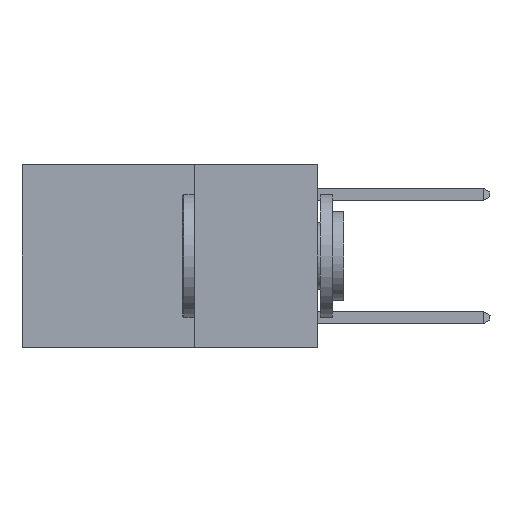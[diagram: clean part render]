
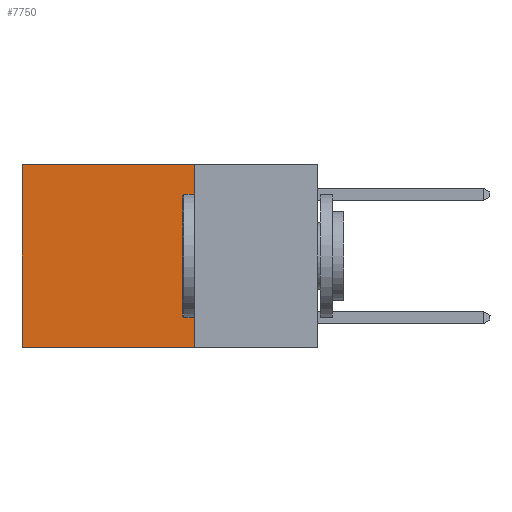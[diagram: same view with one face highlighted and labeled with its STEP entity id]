
A CAD part, left-side view. The second image highlights one B-rep face of the part: STEP entity #7750.
In plain terms, the highlighted planar face has unit normal (-1, 0, 0).
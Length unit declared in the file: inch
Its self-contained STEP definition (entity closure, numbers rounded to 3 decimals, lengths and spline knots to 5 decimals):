
#570 = EDGE_CURVE ( 'NONE', #6980, #10879, #2409, .T. ) ;
#599 = LINE ( 'NONE', #3156, #6562 ) ;
#1293 = DIRECTION ( 'NONE',  ( 0., 0., -1. ) ) ;
#1350 = VECTOR ( 'NONE', #5822, 39.37008 ) ;
#1358 = CARTESIAN_POINT ( 'NONE',  ( 0.2625, 0.25, 0. ) ) ;
#1656 = EDGE_CURVE ( 'NONE', #10879, #11398, #599, .T. ) ;
#2409 = LINE ( 'NONE', #2677, #4765 ) ;
#2545 = AXIS2_PLACEMENT_3D ( 'NONE', #5964, #5924, #1293 ) ;
#2677 = CARTESIAN_POINT ( 'NONE',  ( 0.2625, 0.25, 0. ) ) ;
#2712 = DIRECTION ( 'NONE',  ( 0., 1., 0. ) ) ;
#2843 = EDGE_LOOP ( 'NONE', ( #8108, #5827, #11740, #11342 ) ) ;
#2870 = CARTESIAN_POINT ( 'NONE',  ( 0.2625, 0.25, -0.37 ) ) ;
#3156 = CARTESIAN_POINT ( 'NONE',  ( 0.2625, 0.6, 0. ) ) ;
#3450 = VERTEX_POINT ( 'NONE', #2870 ) ;
#3910 = CARTESIAN_POINT ( 'NONE',  ( 0.2625, 0.6, 0. ) ) ;
#4727 = LINE ( 'NONE', #7664, #1350 ) ;
#4765 = VECTOR ( 'NONE', #2712, 39.37008 ) ;
#5822 = DIRECTION ( 'NONE',  ( 0., 0., -1. ) ) ;
#5827 = ORIENTED_EDGE ( 'NONE', *, *, #9782, .F. ) ;
#5924 = DIRECTION ( 'NONE',  ( 1., 0., 0. ) ) ;
#5964 = CARTESIAN_POINT ( 'NONE',  ( 0.2625, 0.25, 0. ) ) ;
#6031 = PLANE ( 'NONE',  #2545 ) ;
#6421 = CARTESIAN_POINT ( 'NONE',  ( 0.2625, 0.25, -0.37 ) ) ;
#6562 = VECTOR ( 'NONE', #10570, 39.37008 ) ;
#6884 = EDGE_CURVE ( 'NONE', #6980, #3450, #4727, .T. ) ;
#6980 = VERTEX_POINT ( 'NONE', #1358 ) ;
#7345 = DIRECTION ( 'NONE',  ( 0., 1., 0. ) ) ;
#7394 = LINE ( 'NONE', #6421, #8987 ) ;
#7664 = CARTESIAN_POINT ( 'NONE',  ( 0.2625, 0.25, 0. ) ) ;
#7750 = ADVANCED_FACE ( 'NONE', ( #8447 ), #6031, .F. ) ;
#8108 = ORIENTED_EDGE ( 'NONE', *, *, #1656, .T. ) ;
#8447 = FACE_OUTER_BOUND ( 'NONE', #2843, .T. ) ;
#8987 = VECTOR ( 'NONE', #7345, 39.37008 ) ;
#9782 = EDGE_CURVE ( 'NONE', #3450, #11398, #7394, .T. ) ;
#10570 = DIRECTION ( 'NONE',  ( 0., 0., -1. ) ) ;
#10857 = CARTESIAN_POINT ( 'NONE',  ( 0.2625, 0.6, -0.37 ) ) ;
#10879 = VERTEX_POINT ( 'NONE', #3910 ) ;
#11342 = ORIENTED_EDGE ( 'NONE', *, *, #570, .T. ) ;
#11398 = VERTEX_POINT ( 'NONE', #10857 ) ;
#11740 = ORIENTED_EDGE ( 'NONE', *, *, #6884, .F. ) ;
